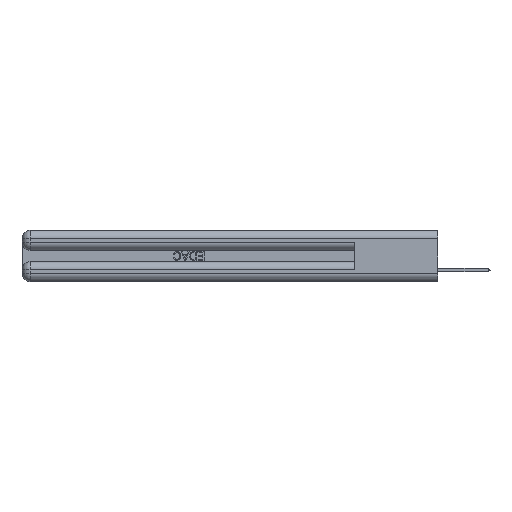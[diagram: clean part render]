
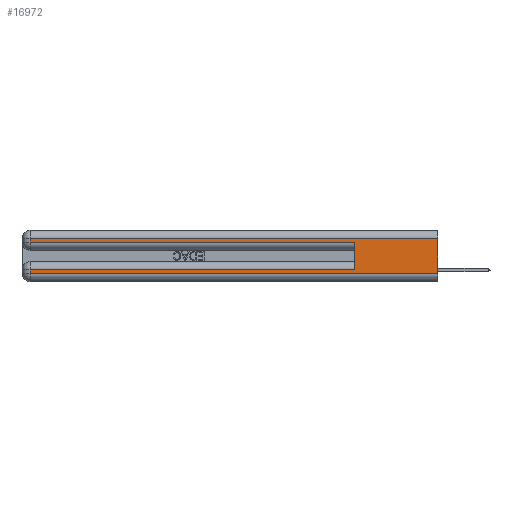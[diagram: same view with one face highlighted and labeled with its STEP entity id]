
A CAD part, left-side view. The second image highlights one B-rep face of the part: STEP entity #16972.
In plain terms, the highlighted planar face has unit normal (-1, 0, 0).
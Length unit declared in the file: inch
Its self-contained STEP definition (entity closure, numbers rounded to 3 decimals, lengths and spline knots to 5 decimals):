
#1204 = LINE ( 'NONE', #39945, #3237 ) ;
#3237 = VECTOR ( 'NONE', #20891, 39.37008 ) ;
#3681 = DIRECTION ( 'NONE',  ( 0., 1., 0. ) ) ;
#4529 = DIRECTION ( 'NONE',  ( 1., 0., 0. ) ) ;
#4856 = LINE ( 'NONE', #8300, #31177 ) ;
#4910 = CARTESIAN_POINT ( 'NONE',  ( 0., 2.94, 0.06 ) ) ;
#5995 = LINE ( 'NONE', #34892, #20844 ) ;
#6106 = EDGE_CURVE ( 'NONE', #30656, #21667, #1204, .T. ) ;
#6127 = AXIS2_PLACEMENT_3D ( 'NONE', #23525, #4529, #8037 ) ;
#6939 = VERTEX_POINT ( 'NONE', #20394 ) ;
#7326 = VERTEX_POINT ( 'NONE', #4910 ) ;
#7335 = DIRECTION ( 'NONE',  ( 0., -1., 0. ) ) ;
#7834 = CARTESIAN_POINT ( 'NONE',  ( 0., 2.94, 0.37 ) ) ;
#8037 = DIRECTION ( 'NONE',  ( 0., 0., -1. ) ) ;
#8300 = CARTESIAN_POINT ( 'NONE',  ( 0., 0., 0.37 ) ) ;
#9373 = CARTESIAN_POINT ( 'NONE',  ( 0., 2.94, 0.285 ) ) ;
#10168 = DIRECTION ( 'NONE',  ( 0., 1., 0. ) ) ;
#10874 = CARTESIAN_POINT ( 'NONE',  ( 0., 2.94, 0.37 ) ) ;
#11206 = VECTOR ( 'NONE', #17647, 39.37008 ) ;
#11221 = VERTEX_POINT ( 'NONE', #38832 ) ;
#11756 = EDGE_CURVE ( 'NONE', #6939, #7326, #20996, .T. ) ;
#12396 = ORIENTED_EDGE ( 'NONE', *, *, #13401, .T. ) ;
#12573 = ORIENTED_EDGE ( 'NONE', *, *, #30574, .F. ) ;
#13401 = EDGE_CURVE ( 'NONE', #11221, #40465, #5995, .T. ) ;
#13520 = ORIENTED_EDGE ( 'NONE', *, *, #20332, .T. ) ;
#14449 = VECTOR ( 'NONE', #7335, 39.37008 ) ;
#14635 = DIRECTION ( 'NONE',  ( 0., 0., -1. ) ) ;
#14987 = LINE ( 'NONE', #22977, #14449 ) ;
#15064 = CARTESIAN_POINT ( 'NONE',  ( 0., 0.6, 0.085 ) ) ;
#15566 = VECTOR ( 'NONE', #39596, 39.37008 ) ;
#15717 = ORIENTED_EDGE ( 'NONE', *, *, #6106, .F. ) ;
#16099 = EDGE_CURVE ( 'NONE', #38939, #21667, #35455, .T. ) ;
#16134 = VECTOR ( 'NONE', #29449, 39.37008 ) ;
#16888 = ORIENTED_EDGE ( 'NONE', *, *, #16099, .T. ) ;
#16960 = CARTESIAN_POINT ( 'NONE',  ( 0., 0., 0.285 ) ) ;
#16972 = ADVANCED_FACE ( 'NONE', ( #29767 ), #27017, .F. ) ;
#17605 = EDGE_CURVE ( 'NONE', #30656, #6939, #32476, .T. ) ;
#17647 = DIRECTION ( 'NONE',  ( 0., 0., -1. ) ) ;
#20332 = EDGE_CURVE ( 'NONE', #7326, #35069, #14987, .T. ) ;
#20394 = CARTESIAN_POINT ( 'NONE',  ( 0., 2.94, 0.085 ) ) ;
#20844 = VECTOR ( 'NONE', #3681, 39.37008 ) ;
#20891 = DIRECTION ( 'NONE',  ( 0., 0., 1. ) ) ;
#20996 = LINE ( 'NONE', #7834, #15566 ) ;
#21098 = ORIENTED_EDGE ( 'NONE', *, *, #11756, .T. ) ;
#21632 = LINE ( 'NONE', #10874, #11206 ) ;
#21667 = VERTEX_POINT ( 'NONE', #25750 ) ;
#21928 = EDGE_LOOP ( 'NONE', ( #12573, #12396, #26628, #16888, #15717, #35179, #21098, #13520 ) ) ;
#22977 = CARTESIAN_POINT ( 'NONE',  ( 0., 0., 0.06 ) ) ;
#23525 = CARTESIAN_POINT ( 'NONE',  ( 0., 0., 0.37 ) ) ;
#25109 = EDGE_CURVE ( 'NONE', #40465, #38939, #21632, .T. ) ;
#25750 = CARTESIAN_POINT ( 'NONE',  ( 0., 0.6, 0.285 ) ) ;
#26628 = ORIENTED_EDGE ( 'NONE', *, *, #25109, .T. ) ;
#27017 = PLANE ( 'NONE',  #6127 ) ;
#29155 = CARTESIAN_POINT ( 'NONE',  ( 0., 0., 0.085 ) ) ;
#29449 = DIRECTION ( 'NONE',  ( 0., -1., 0. ) ) ;
#29767 = FACE_OUTER_BOUND ( 'NONE', #21928, .T. ) ;
#30574 = EDGE_CURVE ( 'NONE', #11221, #35069, #4856, .T. ) ;
#30656 = VERTEX_POINT ( 'NONE', #15064 ) ;
#31177 = VECTOR ( 'NONE', #14635, 39.37008 ) ;
#32476 = LINE ( 'NONE', #29155, #38967 ) ;
#34892 = CARTESIAN_POINT ( 'NONE',  ( 0., 0., 0.31 ) ) ;
#35069 = VERTEX_POINT ( 'NONE', #40168 ) ;
#35179 = ORIENTED_EDGE ( 'NONE', *, *, #17605, .T. ) ;
#35455 = LINE ( 'NONE', #16960, #16134 ) ;
#35735 = CARTESIAN_POINT ( 'NONE',  ( 0., 2.94, 0.31 ) ) ;
#38832 = CARTESIAN_POINT ( 'NONE',  ( 0., 0., 0.31 ) ) ;
#38939 = VERTEX_POINT ( 'NONE', #9373 ) ;
#38967 = VECTOR ( 'NONE', #10168, 39.37008 ) ;
#39596 = DIRECTION ( 'NONE',  ( 0., 0., -1. ) ) ;
#39945 = CARTESIAN_POINT ( 'NONE',  ( 0., 0.6, 0.145 ) ) ;
#40168 = CARTESIAN_POINT ( 'NONE',  ( 0., 0., 0.06 ) ) ;
#40465 = VERTEX_POINT ( 'NONE', #35735 ) ;
